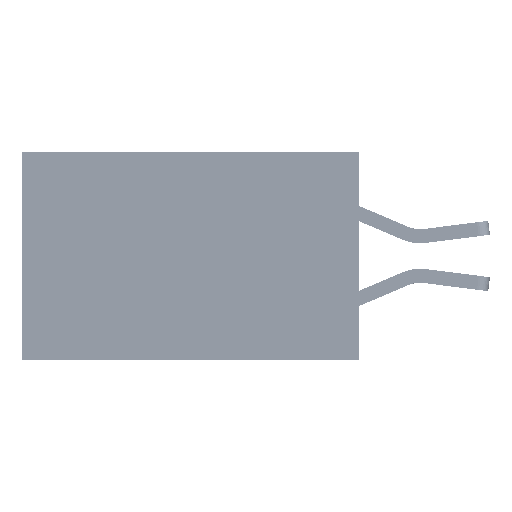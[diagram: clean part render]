
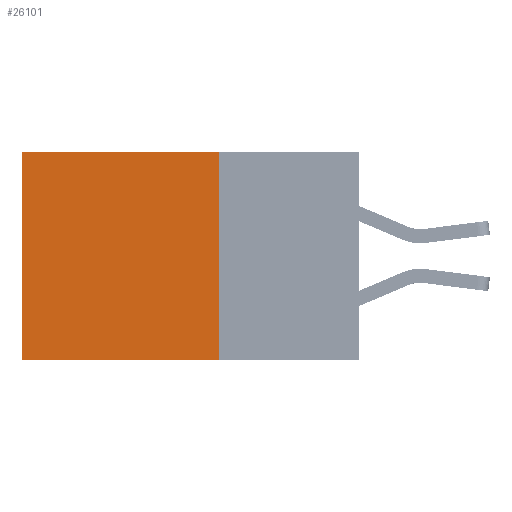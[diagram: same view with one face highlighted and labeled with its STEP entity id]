
A CAD part, left-side view. The second image highlights one B-rep face of the part: STEP entity #26101.
In plain terms, the highlighted planar face has unit normal (-1, 0, 0).
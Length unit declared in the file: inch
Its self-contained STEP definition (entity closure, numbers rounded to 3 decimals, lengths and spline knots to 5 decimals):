
#312 = DIRECTION ( 'NONE',  ( 0., 0., -1. ) ) ;
#1980 = CARTESIAN_POINT ( 'NONE',  ( 0.2875, 0.25, -0.37 ) ) ;
#3729 = VERTEX_POINT ( 'NONE', #39759 ) ;
#4514 = VECTOR ( 'NONE', #41061, 39.37008 ) ;
#7004 = FACE_OUTER_BOUND ( 'NONE', #24419, .T. ) ;
#7670 = VECTOR ( 'NONE', #22939, 39.37008 ) ;
#7711 = CARTESIAN_POINT ( 'NONE',  ( 0.2875, 0.25, -0.37 ) ) ;
#11240 = DIRECTION ( 'NONE',  ( 0., 1., 0. ) ) ;
#11416 = ORIENTED_EDGE ( 'NONE', *, *, #30349, .F. ) ;
#12895 = AXIS2_PLACEMENT_3D ( 'NONE', #41695, #24968, #21440 ) ;
#16402 = EDGE_CURVE ( 'NONE', #3729, #38823, #34583, .T. ) ;
#16568 = LINE ( 'NONE', #37495, #30312 ) ;
#16944 = VECTOR ( 'NONE', #11240, 39.37008 ) ;
#19773 = CARTESIAN_POINT ( 'NONE',  ( 0.2875, 0.6, -0.37 ) ) ;
#21440 = DIRECTION ( 'NONE',  ( 0., 0., -1. ) ) ;
#21595 = PLANE ( 'NONE',  #12895 ) ;
#22939 = DIRECTION ( 'NONE',  ( 0., 0., -1. ) ) ;
#23290 = LINE ( 'NONE', #35146, #16944 ) ;
#24419 = EDGE_LOOP ( 'NONE', ( #31648, #11416, #36580, #29354 ) ) ;
#24968 = DIRECTION ( 'NONE',  ( 1., 0., 0. ) ) ;
#25898 = CARTESIAN_POINT ( 'NONE',  ( 0.2875, 0.25, 0. ) ) ;
#26101 = ADVANCED_FACE ( 'NONE', ( #7004 ), #21595, .F. ) ;
#26343 = VERTEX_POINT ( 'NONE', #19773 ) ;
#27028 = CARTESIAN_POINT ( 'NONE',  ( 0.2875, 0.6, 0. ) ) ;
#27600 = VERTEX_POINT ( 'NONE', #27028 ) ;
#29354 = ORIENTED_EDGE ( 'NONE', *, *, #32397, .T. ) ;
#30312 = VECTOR ( 'NONE', #312, 39.37008 ) ;
#30349 = EDGE_CURVE ( 'NONE', #38823, #26343, #43592, .T. ) ;
#31648 = ORIENTED_EDGE ( 'NONE', *, *, #37014, .T. ) ;
#32397 = EDGE_CURVE ( 'NONE', #3729, #27600, #23290, .T. ) ;
#34583 = LINE ( 'NONE', #25898, #7670 ) ;
#35146 = CARTESIAN_POINT ( 'NONE',  ( 0.2875, 0.25, 0. ) ) ;
#36580 = ORIENTED_EDGE ( 'NONE', *, *, #16402, .F. ) ;
#37014 = EDGE_CURVE ( 'NONE', #27600, #26343, #16568, .T. ) ;
#37495 = CARTESIAN_POINT ( 'NONE',  ( 0.2875, 0.6, 0. ) ) ;
#38823 = VERTEX_POINT ( 'NONE', #1980 ) ;
#39759 = CARTESIAN_POINT ( 'NONE',  ( 0.2875, 0.25, 0. ) ) ;
#41061 = DIRECTION ( 'NONE',  ( 0., 1., 0. ) ) ;
#41695 = CARTESIAN_POINT ( 'NONE',  ( 0.2875, 0.25, 0. ) ) ;
#43592 = LINE ( 'NONE', #7711, #4514 ) ;
